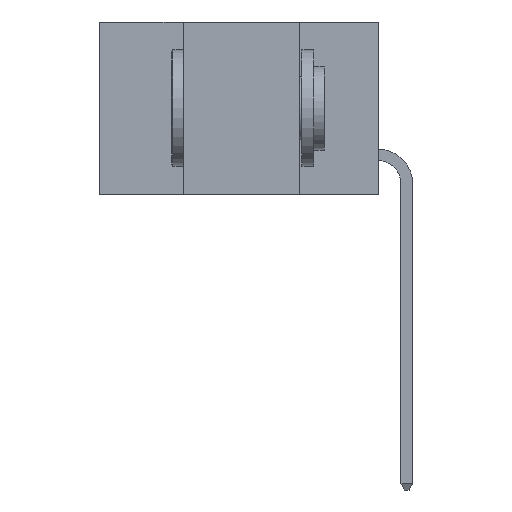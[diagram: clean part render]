
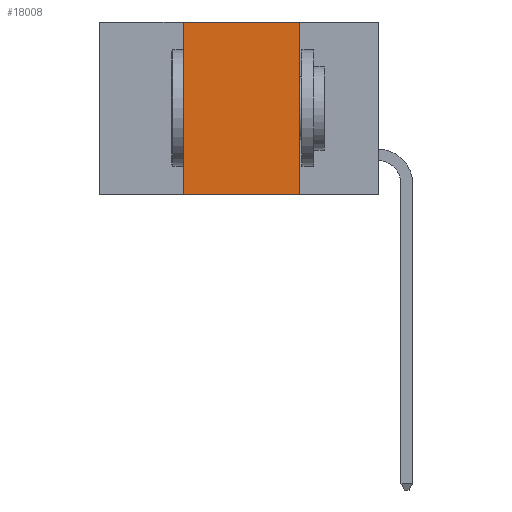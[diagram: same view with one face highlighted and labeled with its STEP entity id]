
A CAD part, left-side view. The second image highlights one B-rep face of the part: STEP entity #18008.
In plain terms, the highlighted planar face has unit normal (-1, 0, 0).
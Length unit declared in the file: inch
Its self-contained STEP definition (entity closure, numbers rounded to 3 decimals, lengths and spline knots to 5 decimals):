
#491 = CARTESIAN_POINT ( 'NONE',  ( 0., 0.42, 0. ) ) ;
#821 = LINE ( 'NONE', #8202, #6226 ) ;
#1174 = VECTOR ( 'NONE', #12898, 39.37008 ) ;
#4461 = LINE ( 'NONE', #17358, #13305 ) ;
#4625 = VECTOR ( 'NONE', #6315, 39.37008 ) ;
#4877 = DIRECTION ( 'NONE',  ( 0., -1., 0. ) ) ;
#5140 = DIRECTION ( 'NONE',  ( 1., 0., 0. ) ) ;
#5480 = EDGE_CURVE ( 'NONE', #19361, #13714, #10513, .T. ) ;
#6226 = VECTOR ( 'NONE', #4877, 39.37008 ) ;
#6315 = DIRECTION ( 'NONE',  ( 0., 0., -1. ) ) ;
#7194 = CARTESIAN_POINT ( 'NONE',  ( 0., 0.42, -0.37 ) ) ;
#7273 = EDGE_CURVE ( 'NONE', #13714, #18674, #4461, .T. ) ;
#8202 = CARTESIAN_POINT ( 'NONE',  ( 0., 0.6, -0.37 ) ) ;
#8325 = AXIS2_PLACEMENT_3D ( 'NONE', #13420, #5140, #16691 ) ;
#8435 = CARTESIAN_POINT ( 'NONE',  ( 0., 0.17, 0. ) ) ;
#8508 = LINE ( 'NONE', #16235, #4625 ) ;
#9154 = DIRECTION ( 'NONE',  ( 0., -1., 0. ) ) ;
#9230 = FACE_OUTER_BOUND ( 'NONE', #11221, .T. ) ;
#9302 = ORIENTED_EDGE ( 'NONE', *, *, #16554, .F. ) ;
#10513 = LINE ( 'NONE', #13247, #1174 ) ;
#10847 = ORIENTED_EDGE ( 'NONE', *, *, #7273, .F. ) ;
#11221 = EDGE_LOOP ( 'NONE', ( #9302, #10847, #15510, #14223 ) ) ;
#11748 = PLANE ( 'NONE',  #8325 ) ;
#12898 = DIRECTION ( 'NONE',  ( 0., 0., 1. ) ) ;
#13247 = CARTESIAN_POINT ( 'NONE',  ( 0., 0.42, -0.37 ) ) ;
#13305 = VECTOR ( 'NONE', #9154, 39.37008 ) ;
#13420 = CARTESIAN_POINT ( 'NONE',  ( 0., 0.6, 0. ) ) ;
#13714 = VERTEX_POINT ( 'NONE', #491 ) ;
#14223 = ORIENTED_EDGE ( 'NONE', *, *, #19743, .T. ) ;
#15510 = ORIENTED_EDGE ( 'NONE', *, *, #5480, .F. ) ;
#16235 = CARTESIAN_POINT ( 'NONE',  ( 0., 0.17, -0.37 ) ) ;
#16554 = EDGE_CURVE ( 'NONE', #18674, #17244, #8508, .T. ) ;
#16691 = DIRECTION ( 'NONE',  ( 0., 0., -1. ) ) ;
#17244 = VERTEX_POINT ( 'NONE', #21052 ) ;
#17358 = CARTESIAN_POINT ( 'NONE',  ( 0., 0.6, 0. ) ) ;
#18008 = ADVANCED_FACE ( 'NONE', ( #9230 ), #11748, .F. ) ;
#18674 = VERTEX_POINT ( 'NONE', #8435 ) ;
#19361 = VERTEX_POINT ( 'NONE', #7194 ) ;
#19743 = EDGE_CURVE ( 'NONE', #19361, #17244, #821, .T. ) ;
#21052 = CARTESIAN_POINT ( 'NONE',  ( 0., 0.17, -0.37 ) ) ;
